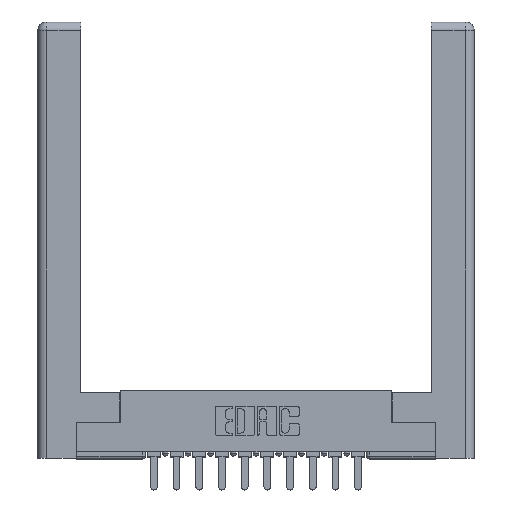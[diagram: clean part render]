
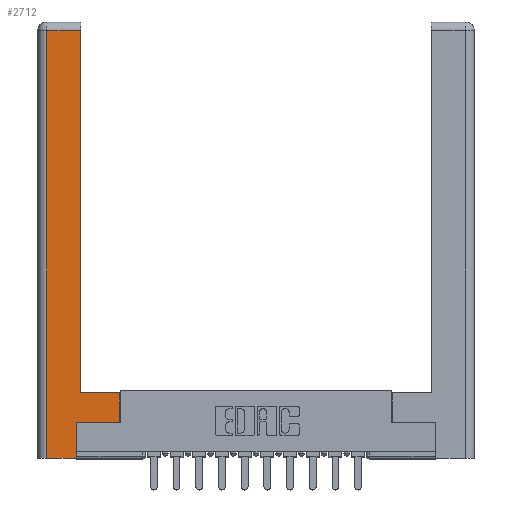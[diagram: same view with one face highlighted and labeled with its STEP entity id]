
A CAD part, top view. The second image highlights one B-rep face of the part: STEP entity #2712.
In plain terms, the highlighted planar face has unit normal (0, 0, 1).
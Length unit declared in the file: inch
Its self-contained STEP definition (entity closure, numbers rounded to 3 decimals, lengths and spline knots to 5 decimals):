
#83 = CARTESIAN_POINT ( 'NONE',  ( 0.295, 0.45, 0. ) ) ;
#723 = ORIENTED_EDGE ( 'NONE', *, *, #8387, .T. ) ;
#1008 = CARTESIAN_POINT ( 'NONE',  ( 0.295, 0.45, 0. ) ) ;
#1149 = EDGE_CURVE ( 'NONE', #11941, #8117, #7422, .T. ) ;
#1312 = CARTESIAN_POINT ( 'NONE',  ( 0.565, 0.245, 0. ) ) ;
#1403 = CARTESIAN_POINT ( 'NONE',  ( 0.265, 0.245, 0. ) ) ;
#1477 = VECTOR ( 'NONE', #14484, 39.37008 ) ;
#1546 = CARTESIAN_POINT ( 'NONE',  ( 0.295, 2.94, 0. ) ) ;
#1629 = LINE ( 'NONE', #1312, #8715 ) ;
#1776 = CARTESIAN_POINT ( 'NONE',  ( 0.265, 0., 0. ) ) ;
#2165 = EDGE_CURVE ( 'NONE', #3676, #3241, #9563, .T. ) ;
#2499 = VECTOR ( 'NONE', #8433, 39.37008 ) ;
#2712 = ADVANCED_FACE ( 'NONE', ( #7183 ), #3277, .F. ) ;
#3241 = VERTEX_POINT ( 'NONE', #5971 ) ;
#3277 = PLANE ( 'NONE',  #5017 ) ;
#3400 = DIRECTION ( 'NONE',  ( -1., 0., 0. ) ) ;
#3517 = CARTESIAN_POINT ( 'NONE',  ( 0., 0., 0. ) ) ;
#3551 = CARTESIAN_POINT ( 'NONE',  ( 0.265, 0., 0. ) ) ;
#3644 = CARTESIAN_POINT ( 'NONE',  ( 0.0615, 2.94, 0. ) ) ;
#3676 = VERTEX_POINT ( 'NONE', #7596 ) ;
#4054 = CARTESIAN_POINT ( 'NONE',  ( 0.265, 0.245, 0. ) ) ;
#4088 = VECTOR ( 'NONE', #6447, 39.37008 ) ;
#4697 = LINE ( 'NONE', #1008, #1477 ) ;
#4822 = CARTESIAN_POINT ( 'NONE',  ( 0.0615, 0., 0. ) ) ;
#4905 = DIRECTION ( 'NONE',  ( 0., 1., 0. ) ) ;
#5017 = AXIS2_PLACEMENT_3D ( 'NONE', #3517, #13383, #10816 ) ;
#5418 = VECTOR ( 'NONE', #12572, 39.37008 ) ;
#5434 = EDGE_CURVE ( 'NONE', #7237, #6033, #6248, .T. ) ;
#5969 = ORIENTED_EDGE ( 'NONE', *, *, #5434, .T. ) ;
#5971 = CARTESIAN_POINT ( 'NONE',  ( 0.0615, 0., 0. ) ) ;
#6033 = VERTEX_POINT ( 'NONE', #1546 ) ;
#6115 = EDGE_CURVE ( 'NONE', #8117, #14944, #1629, .T. ) ;
#6182 = DIRECTION ( 'NONE',  ( 1., 0., 0. ) ) ;
#6248 = LINE ( 'NONE', #8747, #7925 ) ;
#6447 = DIRECTION ( 'NONE',  ( 0., 1., 0. ) ) ;
#7183 = FACE_OUTER_BOUND ( 'NONE', #10583, .T. ) ;
#7237 = VERTEX_POINT ( 'NONE', #83 ) ;
#7269 = CARTESIAN_POINT ( 'NONE',  ( 0.565, 0.45, 0. ) ) ;
#7277 = DIRECTION ( 'NONE',  ( 0., -1., 0. ) ) ;
#7422 = LINE ( 'NONE', #4054, #4088 ) ;
#7596 = CARTESIAN_POINT ( 'NONE',  ( 0.0615, 2.94, 0. ) ) ;
#7925 = VECTOR ( 'NONE', #4905, 39.37008 ) ;
#8117 = VERTEX_POINT ( 'NONE', #1403 ) ;
#8387 = EDGE_CURVE ( 'NONE', #3241, #11941, #15512, .T. ) ;
#8433 = DIRECTION ( 'NONE',  ( 1., 0., 0. ) ) ;
#8715 = VECTOR ( 'NONE', #6182, 39.37008 ) ;
#8747 = CARTESIAN_POINT ( 'NONE',  ( 0.295, 3., 0. ) ) ;
#9559 = EDGE_CURVE ( 'NONE', #10379, #7237, #4697, .T. ) ;
#9563 = LINE ( 'NONE', #4822, #10022 ) ;
#10022 = VECTOR ( 'NONE', #7277, 39.37008 ) ;
#10234 = LINE ( 'NONE', #7269, #5418 ) ;
#10379 = VERTEX_POINT ( 'NONE', #15801 ) ;
#10583 = EDGE_LOOP ( 'NONE', ( #5969, #12576, #11205, #723, #11948, #13501, #12120, #11613 ) ) ;
#10816 = DIRECTION ( 'NONE',  ( -1., 0., 0. ) ) ;
#11006 = LINE ( 'NONE', #3644, #14852 ) ;
#11205 = ORIENTED_EDGE ( 'NONE', *, *, #2165, .T. ) ;
#11613 = ORIENTED_EDGE ( 'NONE', *, *, #9559, .T. ) ;
#11941 = VERTEX_POINT ( 'NONE', #1776 ) ;
#11948 = ORIENTED_EDGE ( 'NONE', *, *, #1149, .T. ) ;
#12120 = ORIENTED_EDGE ( 'NONE', *, *, #12213, .T. ) ;
#12213 = EDGE_CURVE ( 'NONE', #14944, #10379, #10234, .T. ) ;
#12572 = DIRECTION ( 'NONE',  ( 0., 1., 0. ) ) ;
#12576 = ORIENTED_EDGE ( 'NONE', *, *, #15560, .T. ) ;
#13383 = DIRECTION ( 'NONE',  ( 0., 0., -1. ) ) ;
#13501 = ORIENTED_EDGE ( 'NONE', *, *, #6115, .T. ) ;
#14092 = CARTESIAN_POINT ( 'NONE',  ( 0.565, 0.245, 0. ) ) ;
#14484 = DIRECTION ( 'NONE',  ( -1., 0., 0. ) ) ;
#14852 = VECTOR ( 'NONE', #3400, 39.37008 ) ;
#14944 = VERTEX_POINT ( 'NONE', #14092 ) ;
#15512 = LINE ( 'NONE', #3551, #2499 ) ;
#15560 = EDGE_CURVE ( 'NONE', #6033, #3676, #11006, .T. ) ;
#15801 = CARTESIAN_POINT ( 'NONE',  ( 0.565, 0.45, 0. ) ) ;
